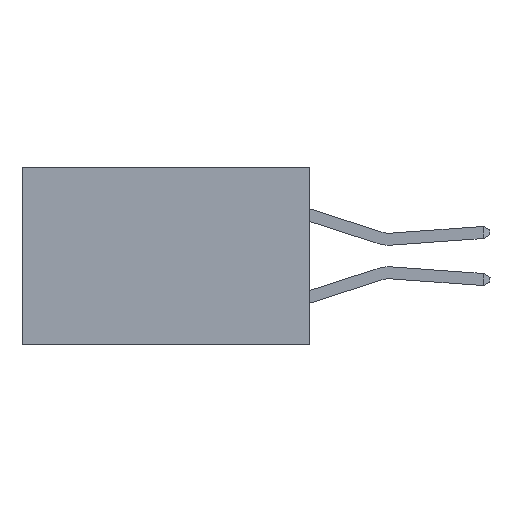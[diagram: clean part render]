
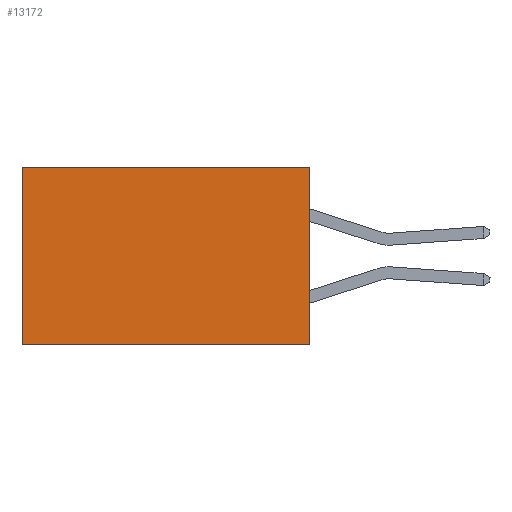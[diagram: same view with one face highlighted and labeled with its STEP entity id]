
A CAD part, left-side view. The second image highlights one B-rep face of the part: STEP entity #13172.
In plain terms, the highlighted planar face has unit normal (-1, 0, 0).
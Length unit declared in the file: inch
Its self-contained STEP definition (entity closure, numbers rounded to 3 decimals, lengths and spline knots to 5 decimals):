
#1862 = EDGE_CURVE ( 'NONE', #8093, #8662, #14655, .T. ) ;
#2742 = CARTESIAN_POINT ( 'NONE',  ( 0.2615, 0., -0.37 ) ) ;
#3774 = ORIENTED_EDGE ( 'NONE', *, *, #7234, .F. ) ;
#3939 = VECTOR ( 'NONE', #16988, 39.37008 ) ;
#4239 = VERTEX_POINT ( 'NONE', #14896 ) ;
#4316 = CARTESIAN_POINT ( 'NONE',  ( 0.2615, 0.6, -0.37 ) ) ;
#4457 = LINE ( 'NONE', #4316, #3939 ) ;
#4511 = CARTESIAN_POINT ( 'NONE',  ( 0.2615, 0., -0.37 ) ) ;
#4602 = DIRECTION ( 'NONE',  ( 1., 0., 0. ) ) ;
#5211 = DIRECTION ( 'NONE',  ( 0., 1., 0. ) ) ;
#6057 = LINE ( 'NONE', #4511, #18165 ) ;
#6107 = DIRECTION ( 'NONE',  ( 0., 0., -1. ) ) ;
#6800 = VERTEX_POINT ( 'NONE', #2742 ) ;
#6965 = CARTESIAN_POINT ( 'NONE',  ( 0.2615, 0., 0. ) ) ;
#7234 = EDGE_CURVE ( 'NONE', #6800, #4239, #7801, .T. ) ;
#7801 = LINE ( 'NONE', #14703, #11552 ) ;
#8093 = VERTEX_POINT ( 'NONE', #6965 ) ;
#8662 = VERTEX_POINT ( 'NONE', #16756 ) ;
#10379 = CARTESIAN_POINT ( 'NONE',  ( 0.2615, 0., 0. ) ) ;
#11552 = VECTOR ( 'NONE', #5211, 39.37008 ) ;
#11864 = DIRECTION ( 'NONE',  ( 0., 1., 0. ) ) ;
#12267 = FACE_OUTER_BOUND ( 'NONE', #16780, .T. ) ;
#12524 = CARTESIAN_POINT ( 'NONE',  ( 0.2615, 0., -0.37 ) ) ;
#13172 = ADVANCED_FACE ( 'NONE', ( #12267 ), #20319, .F. ) ;
#13808 = AXIS2_PLACEMENT_3D ( 'NONE', #12524, #4602, #15701 ) ;
#14377 = ORIENTED_EDGE ( 'NONE', *, *, #1862, .T. ) ;
#14655 = LINE ( 'NONE', #10379, #18319 ) ;
#14703 = CARTESIAN_POINT ( 'NONE',  ( 0.2615, 0., -0.37 ) ) ;
#14870 = ORIENTED_EDGE ( 'NONE', *, *, #15269, .T. ) ;
#14896 = CARTESIAN_POINT ( 'NONE',  ( 0.2615, 0.6, -0.37 ) ) ;
#15269 = EDGE_CURVE ( 'NONE', #8662, #4239, #4457, .T. ) ;
#15701 = DIRECTION ( 'NONE',  ( 0., 0., -1. ) ) ;
#16166 = ORIENTED_EDGE ( 'NONE', *, *, #20285, .F. ) ;
#16756 = CARTESIAN_POINT ( 'NONE',  ( 0.2615, 0.6, 0. ) ) ;
#16780 = EDGE_LOOP ( 'NONE', ( #14870, #3774, #16166, #14377 ) ) ;
#16988 = DIRECTION ( 'NONE',  ( 0., 0., -1. ) ) ;
#18165 = VECTOR ( 'NONE', #6107, 39.37008 ) ;
#18319 = VECTOR ( 'NONE', #11864, 39.37008 ) ;
#20285 = EDGE_CURVE ( 'NONE', #8093, #6800, #6057, .T. ) ;
#20319 = PLANE ( 'NONE',  #13808 ) ;
